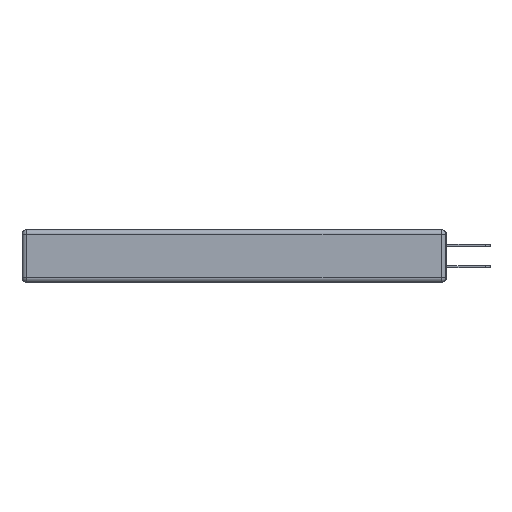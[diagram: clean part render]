
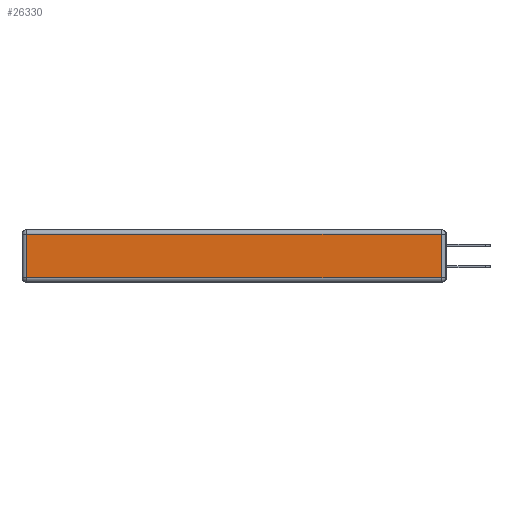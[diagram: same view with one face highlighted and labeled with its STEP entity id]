
A CAD part, left-side view. The second image highlights one B-rep face of the part: STEP entity #26330.
In plain terms, the highlighted planar face has unit normal (-1, 0, 0).
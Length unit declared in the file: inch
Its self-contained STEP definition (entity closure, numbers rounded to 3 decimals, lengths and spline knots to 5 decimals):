
#970 = LINE ( 'NONE', #5803, #27752 ) ;
#2274 = CARTESIAN_POINT ( 'NONE',  ( 0., 2.72, -0.03 ) ) ;
#3171 = CARTESIAN_POINT ( 'NONE',  ( 0., 0., -0.313 ) ) ;
#3856 = VECTOR ( 'NONE', #10936, 39.37008 ) ;
#3858 = EDGE_CURVE ( 'NONE', #25374, #13378, #21449, .T. ) ;
#5036 = DIRECTION ( 'NONE',  ( 0., 0., -1. ) ) ;
#5803 = CARTESIAN_POINT ( 'NONE',  ( 0., 2.75, -0.03 ) ) ;
#6690 = CARTESIAN_POINT ( 'NONE',  ( 0., 0.03, -0.343 ) ) ;
#6943 = VERTEX_POINT ( 'NONE', #2274 ) ;
#7498 = DIRECTION ( 'NONE',  ( -1., 0., 0. ) ) ;
#7798 = EDGE_CURVE ( 'NONE', #6943, #25374, #21985, .T. ) ;
#9938 = LINE ( 'NONE', #6690, #3856 ) ;
#10534 = EDGE_CURVE ( 'NONE', #13378, #26875, #9938, .T. ) ;
#10936 = DIRECTION ( 'NONE',  ( 0., 0., 1. ) ) ;
#11601 = CARTESIAN_POINT ( 'NONE',  ( 0., 0.03, -0.313 ) ) ;
#12027 = CARTESIAN_POINT ( 'NONE',  ( 0., 0., -0.343 ) ) ;
#13378 = VERTEX_POINT ( 'NONE', #11601 ) ;
#13978 = VECTOR ( 'NONE', #18991, 39.37008 ) ;
#14286 = PLANE ( 'NONE',  #16321 ) ;
#15097 = CARTESIAN_POINT ( 'NONE',  ( 0., 2.72, -0.313 ) ) ;
#16051 = CARTESIAN_POINT ( 'NONE',  ( 0., 0.03, -0.03 ) ) ;
#16321 = AXIS2_PLACEMENT_3D ( 'NONE', #12027, #7498, #18372 ) ;
#18290 = EDGE_CURVE ( 'NONE', #26875, #6943, #970, .T. ) ;
#18372 = DIRECTION ( 'NONE',  ( 0., 0., 1. ) ) ;
#18991 = DIRECTION ( 'NONE',  ( 0., -1., 0. ) ) ;
#19062 = ORIENTED_EDGE ( 'NONE', *, *, #7798, .T. ) ;
#20513 = EDGE_LOOP ( 'NONE', ( #24292, #26256, #22918, #19062 ) ) ;
#20977 = DIRECTION ( 'NONE',  ( 0., 1., 0. ) ) ;
#21449 = LINE ( 'NONE', #3171, #13978 ) ;
#21985 = LINE ( 'NONE', #26561, #25013 ) ;
#22854 = FACE_OUTER_BOUND ( 'NONE', #20513, .T. ) ;
#22918 = ORIENTED_EDGE ( 'NONE', *, *, #18290, .T. ) ;
#24292 = ORIENTED_EDGE ( 'NONE', *, *, #3858, .T. ) ;
#25013 = VECTOR ( 'NONE', #5036, 39.37008 ) ;
#25374 = VERTEX_POINT ( 'NONE', #15097 ) ;
#26256 = ORIENTED_EDGE ( 'NONE', *, *, #10534, .T. ) ;
#26330 = ADVANCED_FACE ( 'NONE', ( #22854 ), #14286, .T. ) ;
#26561 = CARTESIAN_POINT ( 'NONE',  ( 0., 2.72, -0.343 ) ) ;
#26875 = VERTEX_POINT ( 'NONE', #16051 ) ;
#27752 = VECTOR ( 'NONE', #20977, 39.37008 ) ;
